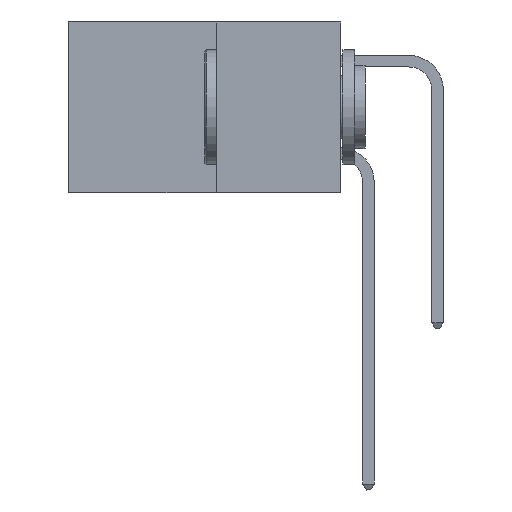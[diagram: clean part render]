
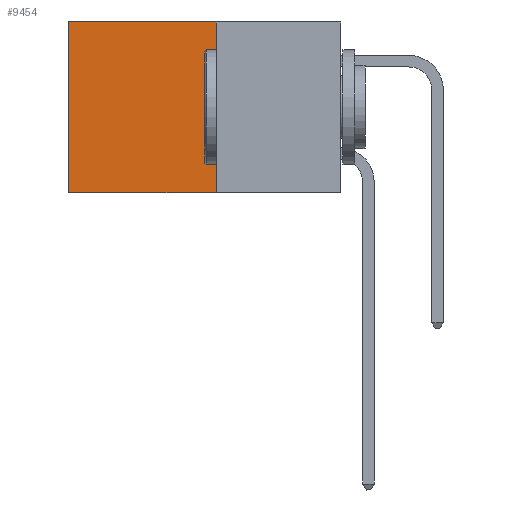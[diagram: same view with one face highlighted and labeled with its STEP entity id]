
A CAD part, left-side view. The second image highlights one B-rep face of the part: STEP entity #9454.
In plain terms, the highlighted planar face has unit normal (-1, 0, 0).
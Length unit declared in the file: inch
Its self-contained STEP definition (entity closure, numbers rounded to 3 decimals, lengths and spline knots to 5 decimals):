
#1239 = LINE ( 'NONE', #6367, #22682 ) ;
#2301 = EDGE_CURVE ( 'NONE', #10400, #33144, #15700, .T. ) ;
#4112 = LINE ( 'NONE', #34584, #18184 ) ;
#5444 = VECTOR ( 'NONE', #28563, 39.37008 ) ;
#6367 = CARTESIAN_POINT ( 'NONE',  ( 0.277, 0.27, -0.37 ) ) ;
#6375 = CARTESIAN_POINT ( 'NONE',  ( 0.277, 0.27, 0. ) ) ;
#6951 = DIRECTION ( 'NONE',  ( 0., 0., -1. ) ) ;
#9126 = VECTOR ( 'NONE', #15578, 39.37008 ) ;
#9415 = CARTESIAN_POINT ( 'NONE',  ( 0.277, 0.59, 0. ) ) ;
#9423 = CARTESIAN_POINT ( 'NONE',  ( 0.277, 0.59, -0.37 ) ) ;
#9454 = ADVANCED_FACE ( 'NONE', ( #30271 ), #16481, .F. ) ;
#10400 = VERTEX_POINT ( 'NONE', #22976 ) ;
#11402 = ORIENTED_EDGE ( 'NONE', *, *, #26250, .F. ) ;
#12987 = LINE ( 'NONE', #6375, #5444 ) ;
#14420 = ORIENTED_EDGE ( 'NONE', *, *, #14664, .T. ) ;
#14610 = CARTESIAN_POINT ( 'NONE',  ( 0.277, 0.27, -0.37 ) ) ;
#14664 = EDGE_CURVE ( 'NONE', #29119, #33144, #4112, .T. ) ;
#15578 = DIRECTION ( 'NONE',  ( 0., 1., 0. ) ) ;
#15700 = LINE ( 'NONE', #14610, #9126 ) ;
#16481 = PLANE ( 'NONE',  #18727 ) ;
#18184 = VECTOR ( 'NONE', #6951, 39.37008 ) ;
#18411 = VERTEX_POINT ( 'NONE', #23448 ) ;
#18727 = AXIS2_PLACEMENT_3D ( 'NONE', #24589, #35689, #19214 ) ;
#19214 = DIRECTION ( 'NONE',  ( 0., 0., -1. ) ) ;
#22682 = VECTOR ( 'NONE', #23001, 39.37008 ) ;
#22976 = CARTESIAN_POINT ( 'NONE',  ( 0.277, 0.27, -0.37 ) ) ;
#23001 = DIRECTION ( 'NONE',  ( 0., 0., -1. ) ) ;
#23448 = CARTESIAN_POINT ( 'NONE',  ( 0.277, 0.27, 0. ) ) ;
#23471 = ORIENTED_EDGE ( 'NONE', *, *, #2301, .F. ) ;
#24589 = CARTESIAN_POINT ( 'NONE',  ( 0.277, 0.27, -0.37 ) ) ;
#25610 = EDGE_LOOP ( 'NONE', ( #14420, #23471, #11402, #30180 ) ) ;
#26250 = EDGE_CURVE ( 'NONE', #18411, #10400, #1239, .T. ) ;
#28563 = DIRECTION ( 'NONE',  ( 0., 1., 0. ) ) ;
#29119 = VERTEX_POINT ( 'NONE', #9415 ) ;
#29731 = EDGE_CURVE ( 'NONE', #18411, #29119, #12987, .T. ) ;
#30180 = ORIENTED_EDGE ( 'NONE', *, *, #29731, .T. ) ;
#30271 = FACE_OUTER_BOUND ( 'NONE', #25610, .T. ) ;
#33144 = VERTEX_POINT ( 'NONE', #9423 ) ;
#34584 = CARTESIAN_POINT ( 'NONE',  ( 0.277, 0.59, -0.37 ) ) ;
#35689 = DIRECTION ( 'NONE',  ( 1., 0., 0. ) ) ;
